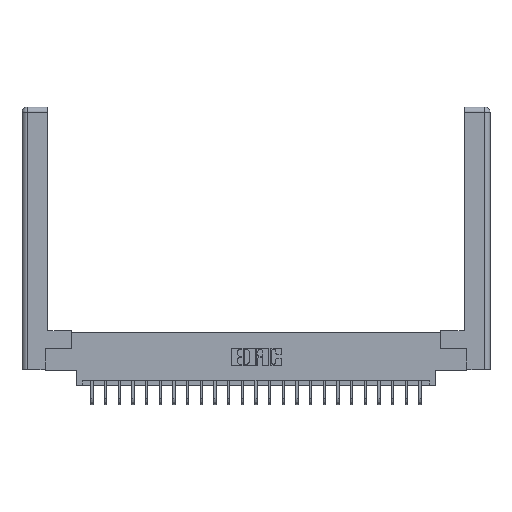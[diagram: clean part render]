
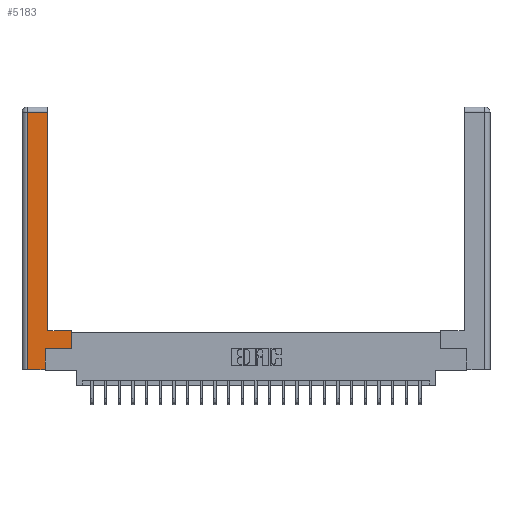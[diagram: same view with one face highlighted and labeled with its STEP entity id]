
A CAD part, top view. The second image highlights one B-rep face of the part: STEP entity #5183.
In plain terms, the highlighted planar face has unit normal (0, 0, 1).
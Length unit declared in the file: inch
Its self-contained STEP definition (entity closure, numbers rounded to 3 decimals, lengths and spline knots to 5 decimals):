
#137 = VECTOR ( 'NONE', #25419, 39.37008 ) ;
#911 = VERTEX_POINT ( 'NONE', #10908 ) ;
#2339 = LINE ( 'NONE', #11070, #10907 ) ;
#2371 = CARTESIAN_POINT ( 'NONE',  ( 0.0615, 0., 0. ) ) ;
#2489 = EDGE_CURVE ( 'NONE', #7842, #3413, #13185, .T. ) ;
#2716 = CARTESIAN_POINT ( 'NONE',  ( 0.295, 2.94, 0. ) ) ;
#3016 = EDGE_CURVE ( 'NONE', #7588, #17821, #2339, .T. ) ;
#3413 = VERTEX_POINT ( 'NONE', #10621 ) ;
#3821 = ORIENTED_EDGE ( 'NONE', *, *, #16389, .T. ) ;
#3851 = ORIENTED_EDGE ( 'NONE', *, *, #14060, .T. ) ;
#4667 = LINE ( 'NONE', #5479, #25516 ) ;
#4732 = ORIENTED_EDGE ( 'NONE', *, *, #2489, .T. ) ;
#4882 = DIRECTION ( 'NONE',  ( 1., 0., 0. ) ) ;
#4947 = LINE ( 'NONE', #15950, #21707 ) ;
#5160 = EDGE_LOOP ( 'NONE', ( #7130, #18878, #15092, #9336, #4732, #3821, #20700, #3851 ) ) ;
#5183 = ADVANCED_FACE ( 'NONE', ( #23482 ), #11391, .F. ) ;
#5479 = CARTESIAN_POINT ( 'NONE',  ( 0.0615, 2.94, 0. ) ) ;
#6350 = CARTESIAN_POINT ( 'NONE',  ( 0.295, 0.45, 0. ) ) ;
#7130 = ORIENTED_EDGE ( 'NONE', *, *, #12004, .T. ) ;
#7181 = VECTOR ( 'NONE', #4882, 39.37008 ) ;
#7313 = CARTESIAN_POINT ( 'NONE',  ( 0.0615, 0., 0. ) ) ;
#7418 = CARTESIAN_POINT ( 'NONE',  ( 0.295, 3., 0. ) ) ;
#7588 = VERTEX_POINT ( 'NONE', #20594 ) ;
#7842 = VERTEX_POINT ( 'NONE', #24363 ) ;
#7927 = VERTEX_POINT ( 'NONE', #2371 ) ;
#8235 = CARTESIAN_POINT ( 'NONE',  ( 0.565, 0.45, 0. ) ) ;
#8764 = VECTOR ( 'NONE', #19276, 39.37008 ) ;
#8953 = DIRECTION ( 'NONE',  ( 0., 1., 0. ) ) ;
#9336 = ORIENTED_EDGE ( 'NONE', *, *, #21152, .T. ) ;
#9736 = EDGE_CURVE ( 'NONE', #14461, #911, #4667, .T. ) ;
#10375 = LINE ( 'NONE', #25021, #7181 ) ;
#10621 = CARTESIAN_POINT ( 'NONE',  ( 0.265, 0.245, 0. ) ) ;
#10907 = VECTOR ( 'NONE', #8953, 39.37008 ) ;
#10908 = CARTESIAN_POINT ( 'NONE',  ( 0.0615, 2.94, 0. ) ) ;
#11070 = CARTESIAN_POINT ( 'NONE',  ( 0.565, 0.45, 0. ) ) ;
#11331 = CARTESIAN_POINT ( 'NONE',  ( 0.565, 0.245, 0. ) ) ;
#11391 = PLANE ( 'NONE',  #22913 ) ;
#11525 = DIRECTION ( 'NONE',  ( -1., 0., 0. ) ) ;
#12004 = EDGE_CURVE ( 'NONE', #22689, #14461, #24469, .T. ) ;
#13185 = LINE ( 'NONE', #20388, #21034 ) ;
#14060 = EDGE_CURVE ( 'NONE', #17821, #22689, #4947, .T. ) ;
#14461 = VERTEX_POINT ( 'NONE', #2716 ) ;
#14549 = EDGE_CURVE ( 'NONE', #911, #7927, #16935, .T. ) ;
#15092 = ORIENTED_EDGE ( 'NONE', *, *, #14549, .T. ) ;
#15951 = DIRECTION ( 'NONE',  ( -1., 0., 0. ) ) ;
#15950 = CARTESIAN_POINT ( 'NONE',  ( 0.295, 0.45, 0. ) ) ;
#16389 = EDGE_CURVE ( 'NONE', #3413, #7588, #19860, .T. ) ;
#16935 = LINE ( 'NONE', #7313, #22625 ) ;
#17588 = DIRECTION ( 'NONE',  ( 0., -1., 0. ) ) ;
#17821 = VERTEX_POINT ( 'NONE', #8235 ) ;
#18878 = ORIENTED_EDGE ( 'NONE', *, *, #9736, .T. ) ;
#19276 = DIRECTION ( 'NONE',  ( 1., 0., 0. ) ) ;
#19343 = CARTESIAN_POINT ( 'NONE',  ( 0., 0., 0. ) ) ;
#19860 = LINE ( 'NONE', #11331, #8764 ) ;
#20388 = CARTESIAN_POINT ( 'NONE',  ( 0.265, 0.245, 0. ) ) ;
#20594 = CARTESIAN_POINT ( 'NONE',  ( 0.565, 0.245, 0. ) ) ;
#20700 = ORIENTED_EDGE ( 'NONE', *, *, #3016, .T. ) ;
#21034 = VECTOR ( 'NONE', #26007, 39.37008 ) ;
#21152 = EDGE_CURVE ( 'NONE', #7927, #7842, #10375, .T. ) ;
#21352 = DIRECTION ( 'NONE',  ( -1., 0., 0. ) ) ;
#21707 = VECTOR ( 'NONE', #11525, 39.37008 ) ;
#22625 = VECTOR ( 'NONE', #17588, 39.37008 ) ;
#22689 = VERTEX_POINT ( 'NONE', #6350 ) ;
#22913 = AXIS2_PLACEMENT_3D ( 'NONE', #19343, #23538, #21352 ) ;
#23482 = FACE_OUTER_BOUND ( 'NONE', #5160, .T. ) ;
#23538 = DIRECTION ( 'NONE',  ( 0., 0., -1. ) ) ;
#24363 = CARTESIAN_POINT ( 'NONE',  ( 0.265, 0., 0. ) ) ;
#24469 = LINE ( 'NONE', #7418, #137 ) ;
#25021 = CARTESIAN_POINT ( 'NONE',  ( 0.265, 0., 0. ) ) ;
#25419 = DIRECTION ( 'NONE',  ( 0., 1., 0. ) ) ;
#25516 = VECTOR ( 'NONE', #15951, 39.37008 ) ;
#26007 = DIRECTION ( 'NONE',  ( 0., 1., 0. ) ) ;
